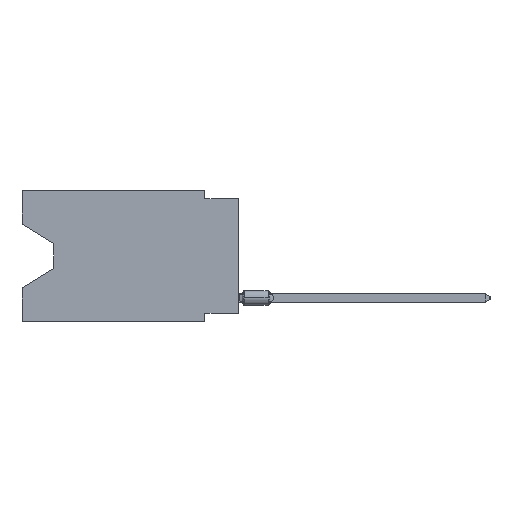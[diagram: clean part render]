
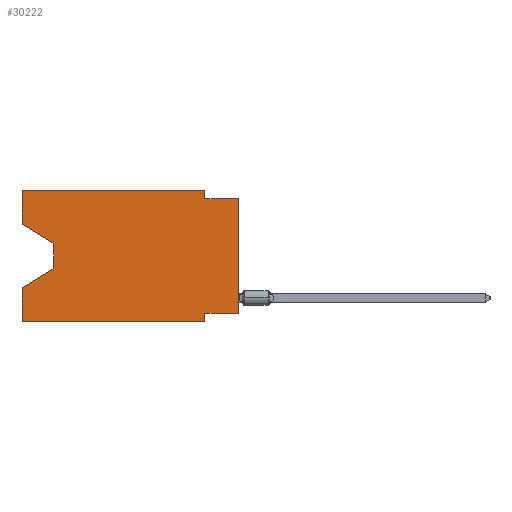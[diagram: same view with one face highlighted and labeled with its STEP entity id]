
A CAD part, left-side view. The second image highlights one B-rep face of the part: STEP entity #30222.
In plain terms, the highlighted planar face has unit normal (-1, 0, 0).
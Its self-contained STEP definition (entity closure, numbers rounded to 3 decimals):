
#808 = CARTESIAN_POINT ( 'NONE',  ( 0., 0., -0.635 ) ) ;
#1779 = ORIENTED_EDGE ( 'NONE', *, *, #10485, .F. ) ;
#2574 = ORIENTED_EDGE ( 'NONE', *, *, #68261, .T. ) ;
#4434 = LINE ( 'NONE', #62024, #45499 ) ;
#4473 = EDGE_CURVE ( 'NONE', #41025, #34923, #54575, .T. ) ;
#6088 = DIRECTION ( 'NONE',  ( 0., -1., 0. ) ) ;
#6457 = EDGE_CURVE ( 'NONE', #26831, #64867, #71967, .T. ) ;
#7006 = DIRECTION ( 'NONE',  ( 0., 0., -1. ) ) ;
#7833 = CARTESIAN_POINT ( 'NONE',  ( 0., 2.54, -0.635 ) ) ;
#7856 = VECTOR ( 'NONE', #6088, 1000. ) ;
#9867 = DIRECTION ( 'NONE',  ( 0., 0., 1. ) ) ;
#10485 = EDGE_CURVE ( 'NONE', #65172, #41025, #50157, .T. ) ;
#10821 = VERTEX_POINT ( 'NONE', #49690 ) ;
#11910 = ORIENTED_EDGE ( 'NONE', *, *, #15360, .T. ) ;
#13193 = CARTESIAN_POINT ( 'NONE',  ( 0., 2.54, 0. ) ) ;
#14162 = EDGE_CURVE ( 'NONE', #10821, #51586, #49877, .T. ) ;
#15360 = EDGE_CURVE ( 'NONE', #65172, #43317, #25776, .T. ) ;
#15873 = CARTESIAN_POINT ( 'NONE',  ( 0., 16.383, -7.36 ) ) ;
#20450 = ORIENTED_EDGE ( 'NONE', *, *, #44390, .F. ) ;
#21976 = LINE ( 'NONE', #49488, #73130 ) ;
#22118 = FACE_OUTER_BOUND ( 'NONE', #49050, .T. ) ;
#22853 = DIRECTION ( 'NONE',  ( 0., 0.855, -0.519 ) ) ;
#23633 = VERTEX_POINT ( 'NONE', #7833 ) ;
#25759 = ORIENTED_EDGE ( 'NONE', *, *, #31051, .F. ) ;
#25776 = LINE ( 'NONE', #60012, #51741 ) ;
#25956 = DIRECTION ( 'NONE',  ( 0., 0., -1. ) ) ;
#26273 = DIRECTION ( 'NONE',  ( 0., 0., -1. ) ) ;
#26831 = VERTEX_POINT ( 'NONE', #30638 ) ;
#26984 = LINE ( 'NONE', #50700, #42837 ) ;
#27767 = PLANE ( 'NONE',  #70411 ) ;
#29002 = CARTESIAN_POINT ( 'NONE',  ( 0., 2.54, -9.271 ) ) ;
#29664 = DIRECTION ( 'NONE',  ( 0., 0., 1. ) ) ;
#30187 = ORIENTED_EDGE ( 'NONE', *, *, #14162, .T. ) ;
#30222 = ADVANCED_FACE ( 'NONE', ( #22118 ), #27767, .F. ) ;
#30638 = CARTESIAN_POINT ( 'NONE',  ( 0., 16.383, -9.906 ) ) ;
#31051 = EDGE_CURVE ( 'NONE', #10821, #56042, #26984, .T. ) ;
#31819 = CARTESIAN_POINT ( 'NONE',  ( 0., 2.54, -9.906 ) ) ;
#32507 = VECTOR ( 'NONE', #22853, 1000. ) ;
#32815 = DIRECTION ( 'NONE',  ( 0., 1., 0. ) ) ;
#34158 = DIRECTION ( 'NONE',  ( 0., -1., 0. ) ) ;
#34923 = VERTEX_POINT ( 'NONE', #31819 ) ;
#35194 = VERTEX_POINT ( 'NONE', #59582 ) ;
#35609 = CARTESIAN_POINT ( 'NONE',  ( 0., 2.54, 0. ) ) ;
#36345 = LINE ( 'NONE', #35609, #40788 ) ;
#37824 = DIRECTION ( 'NONE',  ( 0., -0.855, -0.519 ) ) ;
#40788 = VECTOR ( 'NONE', #7006, 1000. ) ;
#41025 = VERTEX_POINT ( 'NONE', #29002 ) ;
#42562 = VECTOR ( 'NONE', #25956, 1000. ) ;
#42837 = VECTOR ( 'NONE', #72883, 1000. ) ;
#43178 = VECTOR ( 'NONE', #37824, 1000. ) ;
#43197 = EDGE_CURVE ( 'NONE', #35194, #64867, #55637, .T. ) ;
#43317 = VERTEX_POINT ( 'NONE', #61082 ) ;
#43568 = ORIENTED_EDGE ( 'NONE', *, *, #54026, .F. ) ;
#43904 = CARTESIAN_POINT ( 'NONE',  ( 0., 16.383, -9.906 ) ) ;
#44271 = LINE ( 'NONE', #43904, #58289 ) ;
#44390 = EDGE_CURVE ( 'NONE', #56042, #53507, #4434, .T. ) ;
#44713 = CARTESIAN_POINT ( 'NONE',  ( 0., 16.383, 0. ) ) ;
#45499 = VECTOR ( 'NONE', #34158, 1000. ) ;
#46508 = ORIENTED_EDGE ( 'NONE', *, *, #43197, .T. ) ;
#47704 = CARTESIAN_POINT ( 'NONE',  ( 0., 0., -9.271 ) ) ;
#49050 = EDGE_LOOP ( 'NONE', ( #30187, #51677, #46508, #67310, #2574, #59326, #1779, #11910, #73754, #43568, #20450, #25759 ) ) ;
#49103 = CARTESIAN_POINT ( 'NONE',  ( 0., 13.97, -4.013 ) ) ;
#49488 = CARTESIAN_POINT ( 'NONE',  ( 0., 13.97, -4.013 ) ) ;
#49690 = CARTESIAN_POINT ( 'NONE',  ( 0., 16.383, -2.546 ) ) ;
#49877 = LINE ( 'NONE', #50615, #43178 ) ;
#50157 = LINE ( 'NONE', #73084, #71832 ) ;
#50615 = CARTESIAN_POINT ( 'NONE',  ( 0., 16.383, -2.546 ) ) ;
#50700 = CARTESIAN_POINT ( 'NONE',  ( 0., 16.383, 0. ) ) ;
#51288 = CARTESIAN_POINT ( 'NONE',  ( 0., 16.383, 0. ) ) ;
#51586 = VERTEX_POINT ( 'NONE', #49103 ) ;
#51677 = ORIENTED_EDGE ( 'NONE', *, *, #74382, .T. ) ;
#51741 = VECTOR ( 'NONE', #29664, 1000. ) ;
#53507 = VERTEX_POINT ( 'NONE', #13193 ) ;
#54026 = EDGE_CURVE ( 'NONE', #53507, #23633, #36345, .T. ) ;
#54575 = LINE ( 'NONE', #59474, #42562 ) ;
#55637 = LINE ( 'NONE', #56373, #32507 ) ;
#55797 = CARTESIAN_POINT ( 'NONE',  ( 0., 16.383, 0. ) ) ;
#56042 = VERTEX_POINT ( 'NONE', #51288 ) ;
#56237 = DIRECTION ( 'NONE',  ( 0., 0., -1. ) ) ;
#56373 = CARTESIAN_POINT ( 'NONE',  ( 0., 13.97, -5.893 ) ) ;
#57658 = LINE ( 'NONE', #808, #7856 ) ;
#58289 = VECTOR ( 'NONE', #61207, 1000. ) ;
#59326 = ORIENTED_EDGE ( 'NONE', *, *, #4473, .F. ) ;
#59474 = CARTESIAN_POINT ( 'NONE',  ( 0., 2.54, -9.906 ) ) ;
#59582 = CARTESIAN_POINT ( 'NONE',  ( 0., 13.97, -5.893 ) ) ;
#60012 = CARTESIAN_POINT ( 'NONE',  ( 0., 0., 0. ) ) ;
#61082 = CARTESIAN_POINT ( 'NONE',  ( 0., 0., -0.635 ) ) ;
#61207 = DIRECTION ( 'NONE',  ( 0., -1., 0. ) ) ;
#62024 = CARTESIAN_POINT ( 'NONE',  ( 0., 16.383, 0. ) ) ;
#64867 = VERTEX_POINT ( 'NONE', #15873 ) ;
#65172 = VERTEX_POINT ( 'NONE', #47704 ) ;
#66534 = DIRECTION ( 'NONE',  ( 1., 0., 0. ) ) ;
#67310 = ORIENTED_EDGE ( 'NONE', *, *, #6457, .F. ) ;
#68261 = EDGE_CURVE ( 'NONE', #26831, #34923, #44271, .T. ) ;
#70411 = AXIS2_PLACEMENT_3D ( 'NONE', #44713, #66534, #26273 ) ;
#70843 = EDGE_CURVE ( 'NONE', #23633, #43317, #57658, .T. ) ;
#71832 = VECTOR ( 'NONE', #32815, 1000. ) ;
#71967 = LINE ( 'NONE', #55797, #72870 ) ;
#72870 = VECTOR ( 'NONE', #9867, 1000. ) ;
#72883 = DIRECTION ( 'NONE',  ( 0., 0., 1. ) ) ;
#73084 = CARTESIAN_POINT ( 'NONE',  ( 0., 0., -9.271 ) ) ;
#73130 = VECTOR ( 'NONE', #56237, 1000. ) ;
#73754 = ORIENTED_EDGE ( 'NONE', *, *, #70843, .F. ) ;
#74382 = EDGE_CURVE ( 'NONE', #51586, #35194, #21976, .T. ) ;
